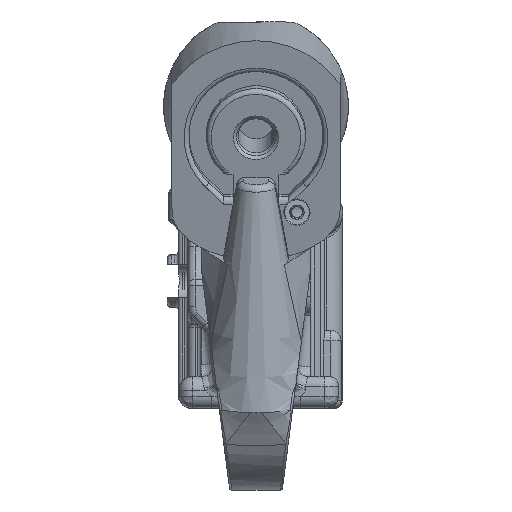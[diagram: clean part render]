
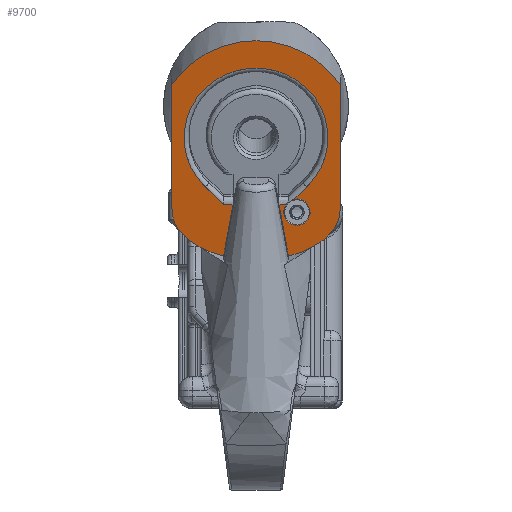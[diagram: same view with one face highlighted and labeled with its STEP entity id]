
A CAD part, front view. The second image highlights one B-rep face of the part: STEP entity #9700.
In plain terms, the highlighted planar face has unit normal (0, -0.966, -0.259).
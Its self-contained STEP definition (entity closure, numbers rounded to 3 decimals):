
#160=ELLIPSE('',#10296,2.847,2.75);
#161=ELLIPSE('',#10297,17.635,10.838);
#164=ELLIPSE('',#10305,2.847,2.75);
#165=ELLIPSE('',#10307,17.635,10.838);
#166=ELLIPSE('',#10309,2.847,2.75);
#167=ELLIPSE('',#10310,17.635,10.838);
#168=ELLIPSE('',#10312,17.635,10.838);
#169=ELLIPSE('',#10313,2.847,2.75);
#324=PLANE('',#10308);
#553=FACE_OUTER_BOUND('',#1112,.T.);
#1112=EDGE_LOOP('',(#6594,#6595,#6596,#6597,#6598,#6599,#6600,#6601,#6602,
#6603,#6604,#6605,#6606,#6607,#6608,#6609,#6610,#6611,#6612));
#1742=B_SPLINE_CURVE_WITH_KNOTS('',3,(#17031,#17032,#17033,#17034),
 .UNSPECIFIED.,.F.,.F.,(4,4),(5.83,5.995),
 .UNSPECIFIED.);
#1985=CIRCLE('',#10301,15.1);
#1986=CIRCLE('',#10311,21.025);
#2415=LINE('',#16941,#3122);
#2422=LINE('',#16973,#3129);
#2426=LINE('',#16985,#3133);
#2429=LINE('',#17006,#3136);
#2432=LINE('',#17021,#3139);
#2433=LINE('',#17025,#3140);
#2434=LINE('',#17029,#3141);
#2435=LINE('',#17036,#3142);
#3122=VECTOR('',#11438,10.);
#3129=VECTOR('',#11455,10.);
#3133=VECTOR('',#11467,10.);
#3136=VECTOR('',#11478,10.);
#3139=VECTOR('',#11487,10.);
#3140=VECTOR('',#11490,10.);
#3141=VECTOR('',#11493,10.);
#3142=VECTOR('',#11496,10.);
#3919=VERTEX_POINT('',#16938);
#3920=VERTEX_POINT('',#16940);
#3922=VERTEX_POINT('',#16950);
#3924=VERTEX_POINT('',#16954);
#3925=VERTEX_POINT('',#16963);
#3926=VERTEX_POINT('',#16965);
#3928=VERTEX_POINT('',#16971);
#3930=VERTEX_POINT('',#16977);
#3932=VERTEX_POINT('',#16983);
#3934=VERTEX_POINT('',#16998);
#3936=VERTEX_POINT('',#17004);
#3937=VERTEX_POINT('',#17013);
#3938=VERTEX_POINT('',#17015);
#3939=VERTEX_POINT('',#17019);
#3940=VERTEX_POINT('',#17022);
#3941=VERTEX_POINT('',#17024);
#3942=VERTEX_POINT('',#17026);
#3943=VERTEX_POINT('',#17028);
#3944=VERTEX_POINT('',#17030);
#4950=EDGE_CURVE('',#3919,#3920,#2415,.T.);
#4955=EDGE_CURVE('',#3924,#3922,#160,.T.);
#4957=EDGE_CURVE('',#3925,#3926,#161,.T.);
#4961=EDGE_CURVE('',#3928,#3919,#2422,.T.);
#4964=EDGE_CURVE('',#3930,#3928,#1985,.T.);
#4967=EDGE_CURVE('',#3932,#3930,#2426,.T.);
#4970=EDGE_CURVE('',#3934,#3932,#164,.T.);
#4973=EDGE_CURVE('',#3936,#3924,#2429,.T.);
#4975=EDGE_CURVE('',#3937,#3938,#165,.T.);
#4977=EDGE_CURVE('',#3922,#3939,#166,.T.);
#4978=EDGE_CURVE('',#3938,#3936,#2432,.T.);
#4979=EDGE_CURVE('',#3940,#3937,#167,.T.);
#4980=EDGE_CURVE('',#3941,#3940,#2433,.T.);
#4981=EDGE_CURVE('',#3942,#3941,#1986,.T.);
#4982=EDGE_CURVE('',#3943,#3942,#2434,.T.);
#4983=EDGE_CURVE('',#3944,#3943,#1742,.T.);
#4984=EDGE_CURVE('',#3926,#3944,#168,.T.);
#4985=EDGE_CURVE('',#3920,#3925,#2435,.T.);
#4986=EDGE_CURVE('',#3939,#3934,#169,.T.);
#6594=ORIENTED_EDGE('',*,*,#4977,.F.);
#6595=ORIENTED_EDGE('',*,*,#4955,.F.);
#6596=ORIENTED_EDGE('',*,*,#4973,.F.);
#6597=ORIENTED_EDGE('',*,*,#4978,.F.);
#6598=ORIENTED_EDGE('',*,*,#4975,.F.);
#6599=ORIENTED_EDGE('',*,*,#4979,.F.);
#6600=ORIENTED_EDGE('',*,*,#4980,.F.);
#6601=ORIENTED_EDGE('',*,*,#4981,.F.);
#6602=ORIENTED_EDGE('',*,*,#4982,.F.);
#6603=ORIENTED_EDGE('',*,*,#4983,.F.);
#6604=ORIENTED_EDGE('',*,*,#4984,.F.);
#6605=ORIENTED_EDGE('',*,*,#4957,.F.);
#6606=ORIENTED_EDGE('',*,*,#4985,.F.);
#6607=ORIENTED_EDGE('',*,*,#4950,.F.);
#6608=ORIENTED_EDGE('',*,*,#4961,.F.);
#6609=ORIENTED_EDGE('',*,*,#4964,.F.);
#6610=ORIENTED_EDGE('',*,*,#4967,.F.);
#6611=ORIENTED_EDGE('',*,*,#4970,.F.);
#6612=ORIENTED_EDGE('',*,*,#4986,.F.);
#9700=ADVANCED_FACE('',(#553),#324,.F.);
#10296=AXIS2_PLACEMENT_3D('',#16956,#11445,#11446);
#10297=AXIS2_PLACEMENT_3D('',#16966,#11448,#11449);
#10301=AXIS2_PLACEMENT_3D('',#16979,#11461,#11462);
#10305=AXIS2_PLACEMENT_3D('',#17000,#11472,#11473);
#10307=AXIS2_PLACEMENT_3D('',#17016,#11480,#11481);
#10308=AXIS2_PLACEMENT_3D('',#17018,#11483,#11484);
#10309=AXIS2_PLACEMENT_3D('',#17020,#11485,#11486);
#10310=AXIS2_PLACEMENT_3D('',#17023,#11488,#11489);
#10311=AXIS2_PLACEMENT_3D('',#17027,#11491,#11492);
#10312=AXIS2_PLACEMENT_3D('',#17035,#11494,#11495);
#10313=AXIS2_PLACEMENT_3D('',#17037,#11497,#11498);
#11438=DIRECTION('',(1.,0.,0.));
#11445=DIRECTION('center_axis',(0.,-0.966,
-0.259));
#11446=DIRECTION('ref_axis',(0.,0.259,-0.966));
#11448=DIRECTION('center_axis',(0.,0.966,
0.259));
#11449=DIRECTION('ref_axis',(1.,0.,0.));
#11455=DIRECTION('',(0.71,0.182,-0.68));
#11461=DIRECTION('center_axis',(0.,-0.966,
-0.259));
#11462=DIRECTION('ref_axis',(0.,-0.259,0.966));
#11467=DIRECTION('',(0.71,-0.182,0.68));
#11472=DIRECTION('center_axis',(0.,-0.966,
-0.259));
#11473=DIRECTION('ref_axis',(0.,0.259,-0.966));
#11478=DIRECTION('',(1.,0.,0.));
#11480=DIRECTION('center_axis',(0.,0.966,
0.259));
#11481=DIRECTION('ref_axis',(1.,0.,0.));
#11483=DIRECTION('center_axis',(0.,0.966,
0.259));
#11484=DIRECTION('ref_axis',(1.,0.,0.));
#11485=DIRECTION('center_axis',(0.,-0.966,
-0.259));
#11486=DIRECTION('ref_axis',(0.,-0.259,0.966));
#11487=DIRECTION('',(-0.174,-0.255,0.951));
#11488=DIRECTION('center_axis',(0.,0.966,
0.259));
#11489=DIRECTION('ref_axis',(1.,0.,0.));
#11490=DIRECTION('',(0.,0.259,-0.966));
#11491=DIRECTION('center_axis',(0.,0.966,
0.259));
#11492=DIRECTION('ref_axis',(-0.839,-0.141,0.526));
#11493=DIRECTION('',(0.,-0.259,0.966));
#11494=DIRECTION('center_axis',(0.,0.966,
0.259));
#11495=DIRECTION('ref_axis',(1.,0.,0.));
#11496=DIRECTION('',(-0.174,0.255,-0.951));
#11497=DIRECTION('center_axis',(0.,-0.966,
-0.259));
#11498=DIRECTION('ref_axis',(0.,-0.259,0.966));
#16938=CARTESIAN_POINT('',(22.875,-133.86,75.107));
#16940=CARTESIAN_POINT('',(24.852,-133.86,75.107));
#16941=CARTESIAN_POINT('',(22.875,-133.86,75.107));
#16950=CARTESIAN_POINT('',(35.512,-133.428,73.497));
#16954=CARTESIAN_POINT('',(36.023,-133.86,75.107));
#16956=CARTESIAN_POINT('Origin',(38.262,-133.432,73.509));
#16963=CARTESIAN_POINT('',(22.875,-130.959,64.282));
#16965=CARTESIAN_POINT('',(18.168,-131.421,66.008));
#16966=CARTESIAN_POINT('Origin',(29.675,-133.547,73.941));
#16971=CARTESIAN_POINT('',(19.049,-134.84,78.768));
#16973=CARTESIAN_POINT('',(21.127,-134.308,76.779));
#16977=CARTESIAN_POINT('',(40.301,-134.84,78.768));
#16979=CARTESIAN_POINT('Origin',(29.675,-137.617,89.13));
#16983=CARTESIAN_POINT('',(37.593,-134.146,76.177));
#16985=CARTESIAN_POINT('',(39.713,-134.69,78.206));
#16998=CARTESIAN_POINT('',(41.012,-133.428,73.497));
#17000=CARTESIAN_POINT('Origin',(38.262,-133.432,73.509));
#17004=CARTESIAN_POINT('',(34.497,-133.86,75.107));
#17006=CARTESIAN_POINT('',(36.475,-133.86,75.107));
#17013=CARTESIAN_POINT('',(41.181,-131.421,66.008));
#17015=CARTESIAN_POINT('',(36.475,-130.959,64.282));
#17016=CARTESIAN_POINT('Origin',(29.675,-133.547,73.941));
#17018=CARTESIAN_POINT('Origin',(29.675,-137.009,86.861));
#17019=CARTESIAN_POINT('',(41.012,-133.425,73.484));
#17020=CARTESIAN_POINT('Origin',(38.262,-133.425,73.484));
#17021=CARTESIAN_POINT('',(33.475,-135.359,80.703));
#17022=CARTESIAN_POINT('',(47.31,-133.547,73.941));
#17023=CARTESIAN_POINT('Origin',(29.675,-133.547,73.941));
#17024=CARTESIAN_POINT('',(47.31,-140.58,100.188));
#17025=CARTESIAN_POINT('',(47.31,-138.795,93.524));
#17026=CARTESIAN_POINT('',(12.04,-140.58,100.188));
#17027=CARTESIAN_POINT('Origin',(29.675,-137.617,89.13));
#17028=CARTESIAN_POINT('',(12.04,-133.741,74.665));
#17029=CARTESIAN_POINT('',(12.04,-135.278,80.401));
#17030=CARTESIAN_POINT('',(12.116,-133.287,72.971));
#17031=CARTESIAN_POINT('Ctrl Pts',(12.116,-133.287,72.971));
#17032=CARTESIAN_POINT('Ctrl Pts',(12.066,-133.443,73.55));
#17033=CARTESIAN_POINT('Ctrl Pts',(12.04,-133.599,74.135));
#17034=CARTESIAN_POINT('Ctrl Pts',(12.04,-133.741,74.665));
#17035=CARTESIAN_POINT('Origin',(29.675,-133.547,73.941));
#17036=CARTESIAN_POINT('',(25.875,-135.359,80.703));
#17037=CARTESIAN_POINT('Origin',(38.262,-133.425,73.484));
